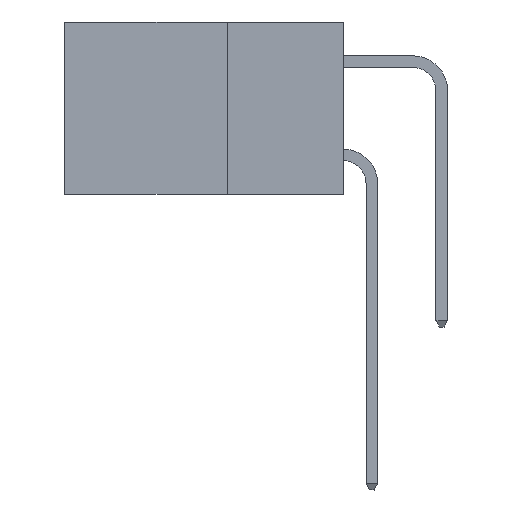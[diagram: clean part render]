
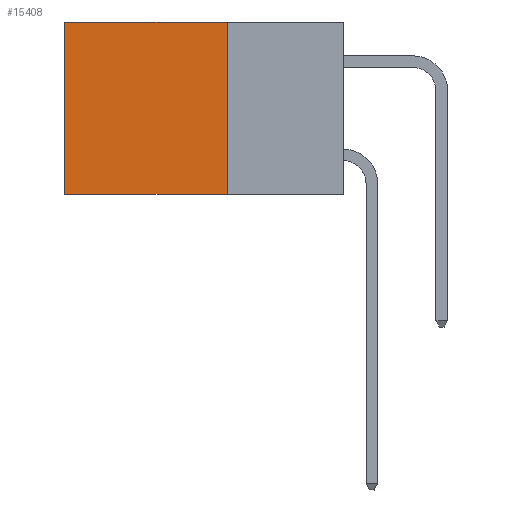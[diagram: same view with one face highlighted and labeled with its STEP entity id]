
A CAD part, left-side view. The second image highlights one B-rep face of the part: STEP entity #15408.
In plain terms, the highlighted planar face has unit normal (-1, 0, 0).
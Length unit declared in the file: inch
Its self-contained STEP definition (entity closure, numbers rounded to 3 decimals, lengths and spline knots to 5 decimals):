
#218 = ORIENTED_EDGE ( 'NONE', *, *, #8702, .T. ) ;
#445 = DIRECTION ( 'NONE',  ( 0., 0., -1. ) ) ;
#454 = DIRECTION ( 'NONE',  ( 0., 1., 0. ) ) ;
#1063 = CARTESIAN_POINT ( 'NONE',  ( 0.298, 0.25, 0. ) ) ;
#1255 = ORIENTED_EDGE ( 'NONE', *, *, #17411, .F. ) ;
#1264 = ORIENTED_EDGE ( 'NONE', *, *, #8299, .F. ) ;
#1379 = VECTOR ( 'NONE', #454, 39.37008 ) ;
#1795 = CARTESIAN_POINT ( 'NONE',  ( 0.298, 0.25, -0.37 ) ) ;
#1811 = DIRECTION ( 'NONE',  ( 0., 1., 0. ) ) ;
#2275 = VECTOR ( 'NONE', #17008, 39.37008 ) ;
#5662 = LINE ( 'NONE', #1063, #2275 ) ;
#6009 = PLANE ( 'NONE',  #18082 ) ;
#6131 = CARTESIAN_POINT ( 'NONE',  ( 0.298, 0.25, 0. ) ) ;
#6356 = CARTESIAN_POINT ( 'NONE',  ( 0.298, 0.6, 0. ) ) ;
#6615 = CARTESIAN_POINT ( 'NONE',  ( 0.298, 0.6, 0. ) ) ;
#7315 = VERTEX_POINT ( 'NONE', #14405 ) ;
#7692 = VECTOR ( 'NONE', #7743, 39.37008 ) ;
#7743 = DIRECTION ( 'NONE',  ( 0., 0., -1. ) ) ;
#8299 = EDGE_CURVE ( 'NONE', #7315, #9308, #9752, .T. ) ;
#8702 = EDGE_CURVE ( 'NONE', #17303, #9308, #17686, .T. ) ;
#9308 = VERTEX_POINT ( 'NONE', #14700 ) ;
#9752 = LINE ( 'NONE', #1795, #1379 ) ;
#10437 = EDGE_CURVE ( 'NONE', #12533, #17303, #18072, .T. ) ;
#10476 = CARTESIAN_POINT ( 'NONE',  ( 0.298, 0.25, 0. ) ) ;
#12034 = ORIENTED_EDGE ( 'NONE', *, *, #10437, .T. ) ;
#12533 = VERTEX_POINT ( 'NONE', #18722 ) ;
#14201 = VECTOR ( 'NONE', #1811, 39.37008 ) ;
#14405 = CARTESIAN_POINT ( 'NONE',  ( 0.298, 0.25, -0.37 ) ) ;
#14700 = CARTESIAN_POINT ( 'NONE',  ( 0.298, 0.6, -0.37 ) ) ;
#15129 = EDGE_LOOP ( 'NONE', ( #218, #1264, #1255, #12034 ) ) ;
#15408 = ADVANCED_FACE ( 'NONE', ( #15502 ), #6009, .F. ) ;
#15502 = FACE_OUTER_BOUND ( 'NONE', #15129, .T. ) ;
#17008 = DIRECTION ( 'NONE',  ( 0., 0., -1. ) ) ;
#17303 = VERTEX_POINT ( 'NONE', #6615 ) ;
#17411 = EDGE_CURVE ( 'NONE', #12533, #7315, #5662, .T. ) ;
#17686 = LINE ( 'NONE', #6356, #7692 ) ;
#17728 = DIRECTION ( 'NONE',  ( 1., 0., 0. ) ) ;
#18072 = LINE ( 'NONE', #10476, #14201 ) ;
#18082 = AXIS2_PLACEMENT_3D ( 'NONE', #6131, #17728, #445 ) ;
#18722 = CARTESIAN_POINT ( 'NONE',  ( 0.298, 0.25, 0. ) ) ;
